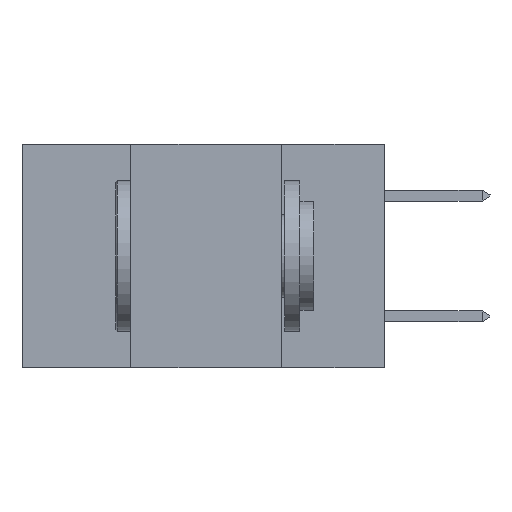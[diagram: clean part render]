
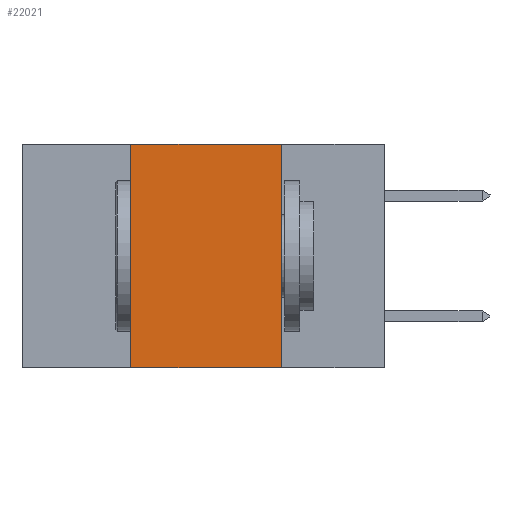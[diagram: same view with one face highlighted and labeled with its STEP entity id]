
A CAD part, left-side view. The second image highlights one B-rep face of the part: STEP entity #22021.
In plain terms, the highlighted planar face has unit normal (-1, 0, 0).
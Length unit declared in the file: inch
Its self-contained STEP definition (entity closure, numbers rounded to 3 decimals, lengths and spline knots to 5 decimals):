
#796 = LINE ( 'NONE', #1260, #11899 ) ;
#1160 = CARTESIAN_POINT ( 'NONE',  ( 0., 0.42, 0. ) ) ;
#1260 = CARTESIAN_POINT ( 'NONE',  ( 0., 0.6, 0. ) ) ;
#1355 = AXIS2_PLACEMENT_3D ( 'NONE', #26472, #24540, #12278 ) ;
#3295 = DIRECTION ( 'NONE',  ( 0., -1., 0. ) ) ;
#5810 = CARTESIAN_POINT ( 'NONE',  ( 0., 0.17, 0. ) ) ;
#6670 = FACE_OUTER_BOUND ( 'NONE', #13408, .T. ) ;
#7002 = LINE ( 'NONE', #1160, #17415 ) ;
#7338 = ORIENTED_EDGE ( 'NONE', *, *, #16018, .F. ) ;
#8066 = PLANE ( 'NONE',  #1355 ) ;
#8626 = ORIENTED_EDGE ( 'NONE', *, *, #26556, .T. ) ;
#8897 = CARTESIAN_POINT ( 'NONE',  ( 0., 0.17, -0.37 ) ) ;
#10415 = EDGE_CURVE ( 'NONE', #10943, #23629, #7002, .T. ) ;
#10451 = EDGE_CURVE ( 'NONE', #23629, #22454, #796, .T. ) ;
#10943 = VERTEX_POINT ( 'NONE', #21856 ) ;
#11639 = DIRECTION ( 'NONE',  ( 0., -1., 0. ) ) ;
#11899 = VECTOR ( 'NONE', #11639, 39.37008 ) ;
#12278 = DIRECTION ( 'NONE',  ( 0., 0., -1. ) ) ;
#13016 = VECTOR ( 'NONE', #16156, 39.37008 ) ;
#13408 = EDGE_LOOP ( 'NONE', ( #7338, #19018, #24414, #8626 ) ) ;
#13598 = VERTEX_POINT ( 'NONE', #8897 ) ;
#13674 = LINE ( 'NONE', #5810, #13016 ) ;
#13678 = CARTESIAN_POINT ( 'NONE',  ( 0., 0.6, -0.37 ) ) ;
#16018 = EDGE_CURVE ( 'NONE', #22454, #13598, #13674, .T. ) ;
#16156 = DIRECTION ( 'NONE',  ( 0., 0., -1. ) ) ;
#17398 = LINE ( 'NONE', #13678, #22175 ) ;
#17415 = VECTOR ( 'NONE', #25860, 39.37008 ) ;
#19018 = ORIENTED_EDGE ( 'NONE', *, *, #10451, .F. ) ;
#21856 = CARTESIAN_POINT ( 'NONE',  ( 0., 0.42, -0.37 ) ) ;
#22021 = ADVANCED_FACE ( 'NONE', ( #6670 ), #8066, .F. ) ;
#22175 = VECTOR ( 'NONE', #3295, 39.37008 ) ;
#22318 = CARTESIAN_POINT ( 'NONE',  ( 0., 0.42, 0. ) ) ;
#22454 = VERTEX_POINT ( 'NONE', #25919 ) ;
#23629 = VERTEX_POINT ( 'NONE', #22318 ) ;
#24414 = ORIENTED_EDGE ( 'NONE', *, *, #10415, .F. ) ;
#24540 = DIRECTION ( 'NONE',  ( 1., 0., 0. ) ) ;
#25860 = DIRECTION ( 'NONE',  ( 0., 0., 1. ) ) ;
#25919 = CARTESIAN_POINT ( 'NONE',  ( 0., 0.17, 0. ) ) ;
#26472 = CARTESIAN_POINT ( 'NONE',  ( 0., 0.6, 0. ) ) ;
#26556 = EDGE_CURVE ( 'NONE', #10943, #13598, #17398, .T. ) ;
